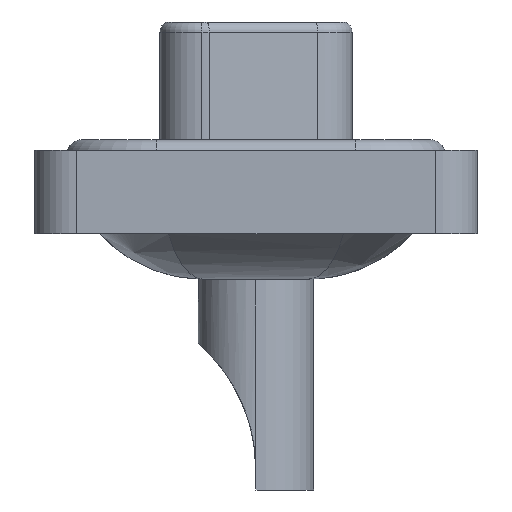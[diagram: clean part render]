
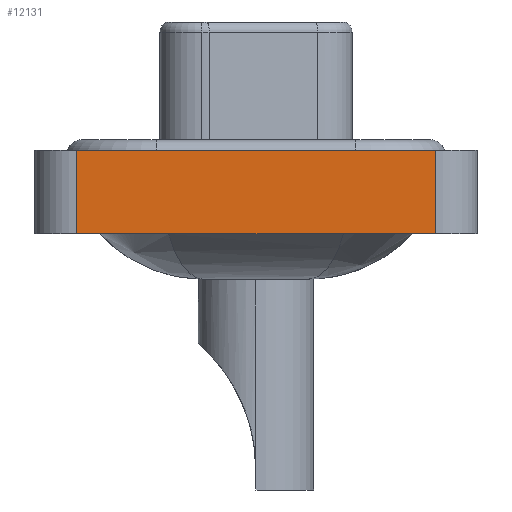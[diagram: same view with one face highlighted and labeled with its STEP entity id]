
A CAD part, left-side view. The second image highlights one B-rep face of the part: STEP entity #12131.
In plain terms, the highlighted planar face has unit normal (-1, 0, 0).
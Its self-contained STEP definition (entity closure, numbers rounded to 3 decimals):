
#1947 = CARTESIAN_POINT ( 'NONE',  ( -7.3, 8.55, -3.6 ) ) ;
#2084 = PLANE ( 'NONE',  #11880 ) ;
#2143 = VERTEX_POINT ( 'NONE', #7426 ) ;
#2277 = VECTOR ( 'NONE', #8739, 1000. ) ;
#2335 = DIRECTION ( 'NONE',  ( 0., -1., 0. ) ) ;
#2716 = LINE ( 'NONE', #7823, #12872 ) ;
#2748 = EDGE_LOOP ( 'NONE', ( #8870, #10060, #10035, #5617 ) ) ;
#3673 = CARTESIAN_POINT ( 'NONE',  ( -7.3, -8.55, -3.6 ) ) ;
#4368 = LINE ( 'NONE', #12006, #4655 ) ;
#4655 = VECTOR ( 'NONE', #15501, 1000. ) ;
#4701 = CARTESIAN_POINT ( 'NONE',  ( -7.3, 8.55, -3.6 ) ) ;
#5590 = EDGE_CURVE ( 'NONE', #6673, #2143, #2716, .T. ) ;
#5617 = ORIENTED_EDGE ( 'NONE', *, *, #11956, .T. ) ;
#5768 = VERTEX_POINT ( 'NONE', #1947 ) ;
#6673 = VERTEX_POINT ( 'NONE', #9713 ) ;
#7372 = DIRECTION ( 'NONE',  ( -1., 0., 0. ) ) ;
#7426 = CARTESIAN_POINT ( 'NONE',  ( -7.3, -8.55, 0.4 ) ) ;
#7823 = CARTESIAN_POINT ( 'NONE',  ( -7.3, -8.55, -3.6 ) ) ;
#8464 = FACE_OUTER_BOUND ( 'NONE', #2748, .T. ) ;
#8548 = DIRECTION ( 'NONE',  ( 0., 0., 1. ) ) ;
#8739 = DIRECTION ( 'NONE',  ( 0., 0., 1. ) ) ;
#8870 = ORIENTED_EDGE ( 'NONE', *, *, #5590, .T. ) ;
#9335 = DIRECTION ( 'NONE',  ( 0., 0., 1. ) ) ;
#9713 = CARTESIAN_POINT ( 'NONE',  ( -7.3, -8.55, -3.6 ) ) ;
#10035 = ORIENTED_EDGE ( 'NONE', *, *, #12937, .F. ) ;
#10060 = ORIENTED_EDGE ( 'NONE', *, *, #14695, .F. ) ;
#10415 = CARTESIAN_POINT ( 'NONE',  ( -7.3, 8.55, 0.4 ) ) ;
#11411 = LINE ( 'NONE', #4701, #2277 ) ;
#11880 = AXIS2_PLACEMENT_3D ( 'NONE', #3673, #7372, #8548 ) ;
#11956 = EDGE_CURVE ( 'NONE', #5768, #6673, #4368, .T. ) ;
#12006 = CARTESIAN_POINT ( 'NONE',  ( -7.3, -8.55, -3.6 ) ) ;
#12131 = ADVANCED_FACE ( 'NONE', ( #8464 ), #2084, .T. ) ;
#12680 = VERTEX_POINT ( 'NONE', #10415 ) ;
#12872 = VECTOR ( 'NONE', #9335, 1000. ) ;
#12937 = EDGE_CURVE ( 'NONE', #5768, #12680, #11411, .T. ) ;
#14695 = EDGE_CURVE ( 'NONE', #12680, #2143, #14993, .T. ) ;
#14993 = LINE ( 'NONE', #16547, #16386 ) ;
#15501 = DIRECTION ( 'NONE',  ( 0., -1., 0. ) ) ;
#16386 = VECTOR ( 'NONE', #2335, 1000. ) ;
#16547 = CARTESIAN_POINT ( 'NONE',  ( -7.3, -8.55, 0.4 ) ) ;
